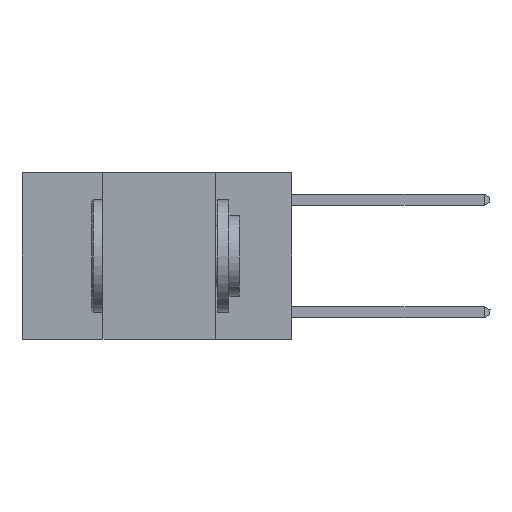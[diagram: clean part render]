
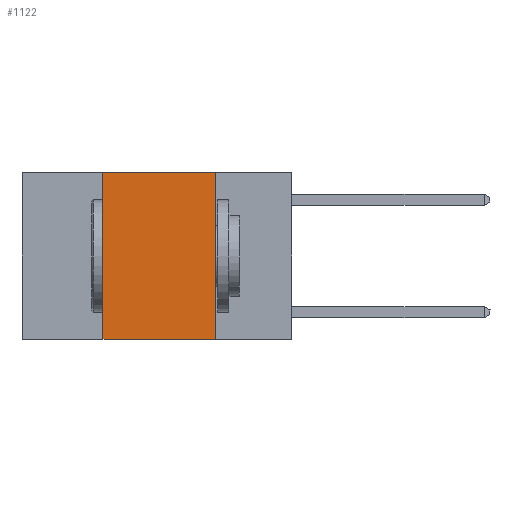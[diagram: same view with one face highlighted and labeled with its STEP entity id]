
A CAD part, left-side view. The second image highlights one B-rep face of the part: STEP entity #1122.
In plain terms, the highlighted planar face has unit normal (-1, 0, 0).
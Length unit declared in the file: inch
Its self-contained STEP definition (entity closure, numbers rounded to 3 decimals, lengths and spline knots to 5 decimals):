
#1122 = ADVANCED_FACE ( 'NONE', ( #8436 ), #14905, .F. ) ;
#1418 = CARTESIAN_POINT ( 'NONE',  ( 0., 0.6, -0.37 ) ) ;
#2506 = CARTESIAN_POINT ( 'NONE',  ( 0., 0.17, 0. ) ) ;
#2751 = VECTOR ( 'NONE', #5425, 39.37008 ) ;
#3121 = CARTESIAN_POINT ( 'NONE',  ( 0., 0.17, -0.37 ) ) ;
#3492 = DIRECTION ( 'NONE',  ( 0., 0., 1. ) ) ;
#4267 = AXIS2_PLACEMENT_3D ( 'NONE', #14811, #14695, #14652 ) ;
#4736 = EDGE_CURVE ( 'NONE', #12260, #9771, #5725, .T. ) ;
#5425 = DIRECTION ( 'NONE',  ( 0., 0., -1. ) ) ;
#5725 = LINE ( 'NONE', #10634, #13647 ) ;
#5762 = EDGE_CURVE ( 'NONE', #9771, #7403, #18608, .T. ) ;
#7403 = VERTEX_POINT ( 'NONE', #3121 ) ;
#7404 = EDGE_CURVE ( 'NONE', #7702, #7403, #12478, .T. ) ;
#7421 = LINE ( 'NONE', #16878, #18688 ) ;
#7702 = VERTEX_POINT ( 'NONE', #11313 ) ;
#8436 = FACE_OUTER_BOUND ( 'NONE', #12464, .T. ) ;
#9771 = VERTEX_POINT ( 'NONE', #2506 ) ;
#10634 = CARTESIAN_POINT ( 'NONE',  ( 0., 0.6, 0. ) ) ;
#10705 = ORIENTED_EDGE ( 'NONE', *, *, #16710, .F. ) ;
#11313 = CARTESIAN_POINT ( 'NONE',  ( 0., 0.42, -0.37 ) ) ;
#11394 = CARTESIAN_POINT ( 'NONE',  ( 0., 0.17, 0. ) ) ;
#11684 = ORIENTED_EDGE ( 'NONE', *, *, #5762, .F. ) ;
#12260 = VERTEX_POINT ( 'NONE', #17763 ) ;
#12464 = EDGE_LOOP ( 'NONE', ( #11684, #18454, #10705, #16239 ) ) ;
#12478 = LINE ( 'NONE', #1418, #15896 ) ;
#13647 = VECTOR ( 'NONE', #15062, 39.37008 ) ;
#14652 = DIRECTION ( 'NONE',  ( 0., 0., -1. ) ) ;
#14695 = DIRECTION ( 'NONE',  ( 1., 0., 0. ) ) ;
#14811 = CARTESIAN_POINT ( 'NONE',  ( 0., 0.6, 0. ) ) ;
#14905 = PLANE ( 'NONE',  #4267 ) ;
#15062 = DIRECTION ( 'NONE',  ( 0., -1., 0. ) ) ;
#15896 = VECTOR ( 'NONE', #18038, 39.37008 ) ;
#16239 = ORIENTED_EDGE ( 'NONE', *, *, #7404, .T. ) ;
#16710 = EDGE_CURVE ( 'NONE', #7702, #12260, #7421, .T. ) ;
#16878 = CARTESIAN_POINT ( 'NONE',  ( 0., 0.42, 0. ) ) ;
#17763 = CARTESIAN_POINT ( 'NONE',  ( 0., 0.42, 0. ) ) ;
#18038 = DIRECTION ( 'NONE',  ( 0., -1., 0. ) ) ;
#18454 = ORIENTED_EDGE ( 'NONE', *, *, #4736, .F. ) ;
#18608 = LINE ( 'NONE', #11394, #2751 ) ;
#18688 = VECTOR ( 'NONE', #3492, 39.37008 ) ;
